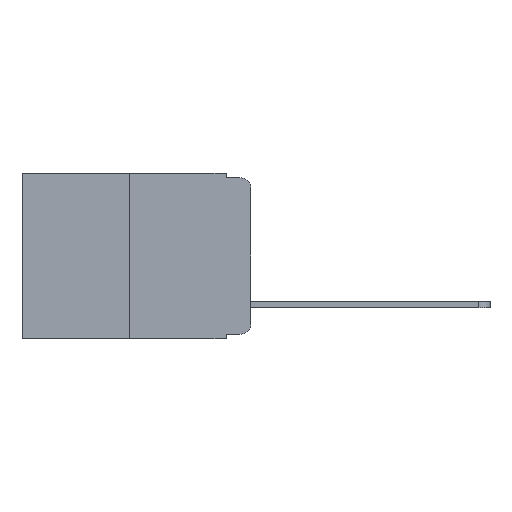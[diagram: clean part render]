
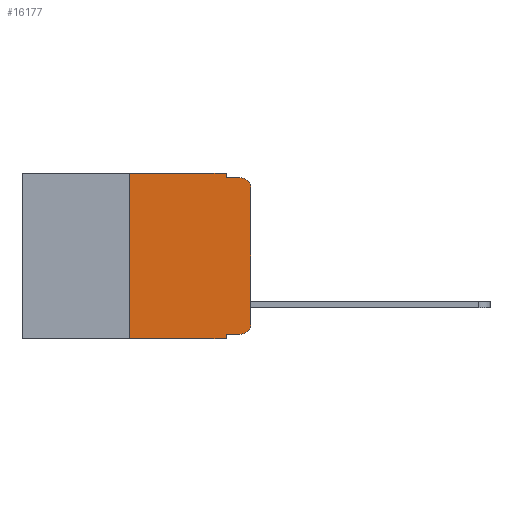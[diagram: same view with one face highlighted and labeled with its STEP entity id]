
A CAD part, left-side view. The second image highlights one B-rep face of the part: STEP entity #16177.
In plain terms, the highlighted planar face has unit normal (-1, 0, 0).
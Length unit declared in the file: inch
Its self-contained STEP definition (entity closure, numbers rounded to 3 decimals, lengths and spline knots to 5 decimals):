
#381 = DIRECTION ( 'NONE',  ( 0., -1., 0. ) ) ;
#1298 = LINE ( 'NONE', #11117, #1922 ) ;
#1876 = VECTOR ( 'NONE', #25471, 39.37008 ) ;
#1922 = VECTOR ( 'NONE', #12966, 39.37008 ) ;
#3066 = DIRECTION ( 'NONE',  ( 0., 0., -1. ) ) ;
#3145 = CARTESIAN_POINT ( 'NONE',  ( 0., 0.02, -0.313 ) ) ;
#3162 = ORIENTED_EDGE ( 'NONE', *, *, #18410, .T. ) ;
#3527 = CARTESIAN_POINT ( 'NONE',  ( 0., 0.473, 0. ) ) ;
#3782 = CARTESIAN_POINT ( 'NONE',  ( 0., 0.051, -0.01 ) ) ;
#4241 = ORIENTED_EDGE ( 'NONE', *, *, #22553, .F. ) ;
#4274 = CARTESIAN_POINT ( 'NONE',  ( 0., 0., -0.313 ) ) ;
#4508 = VERTEX_POINT ( 'NONE', #16672 ) ;
#5679 = LINE ( 'NONE', #9997, #5983 ) ;
#5983 = VECTOR ( 'NONE', #12033, 39.37008 ) ;
#6054 = LINE ( 'NONE', #16431, #22130 ) ;
#6550 = ORIENTED_EDGE ( 'NONE', *, *, #18586, .F. ) ;
#6836 = EDGE_CURVE ( 'NONE', #21819, #19800, #9442, .T. ) ;
#7178 = CARTESIAN_POINT ( 'NONE',  ( 0., 0.02, -0.01 ) ) ;
#7381 = VERTEX_POINT ( 'NONE', #7178 ) ;
#7676 = VERTEX_POINT ( 'NONE', #13423 ) ;
#7685 = VERTEX_POINT ( 'NONE', #25169 ) ;
#7914 = EDGE_LOOP ( 'NONE', ( #20988, #16805, #23745, #6550, #9480, #4241, #24558, #19415, #18828, #3162 ) ) ;
#8549 = CIRCLE ( 'NONE', #22609, 0.02 ) ;
#8832 = CARTESIAN_POINT ( 'NONE',  ( 0., 0.02, -0.03 ) ) ;
#9442 = LINE ( 'NONE', #25559, #26167 ) ;
#9480 = ORIENTED_EDGE ( 'NONE', *, *, #9622, .F. ) ;
#9574 = CARTESIAN_POINT ( 'NONE',  ( 0., 0.051, 0. ) ) ;
#9622 = EDGE_CURVE ( 'NONE', #22339, #7676, #6054, .T. ) ;
#9995 = EDGE_CURVE ( 'NONE', #4508, #7685, #1298, .T. ) ;
#9997 = CARTESIAN_POINT ( 'NONE',  ( 0., 0., 0. ) ) ;
#10143 = EDGE_CURVE ( 'NONE', #10325, #7381, #13927, .T. ) ;
#10325 = VERTEX_POINT ( 'NONE', #11975 ) ;
#10834 = DIRECTION ( 'NONE',  ( 0., 0., -1. ) ) ;
#11117 = CARTESIAN_POINT ( 'NONE',  ( 0., 0.051, -0.333 ) ) ;
#11201 = CARTESIAN_POINT ( 'NONE',  ( 0., 0.25, 0. ) ) ;
#11374 = LINE ( 'NONE', #9574, #1876 ) ;
#11426 = AXIS2_PLACEMENT_3D ( 'NONE', #3527, #21588, #15346 ) ;
#11616 = DIRECTION ( 'NONE',  ( 0., -1., 0. ) ) ;
#11975 = CARTESIAN_POINT ( 'NONE',  ( 0., 0., -0.03 ) ) ;
#12033 = DIRECTION ( 'NONE',  ( 0., 0., 1. ) ) ;
#12966 = DIRECTION ( 'NONE',  ( 0., -1., 0. ) ) ;
#12997 = AXIS2_PLACEMENT_3D ( 'NONE', #8832, #22926, #10834 ) ;
#13423 = CARTESIAN_POINT ( 'NONE',  ( 0., 0.051, 0. ) ) ;
#13927 = CIRCLE ( 'NONE', #12997, 0.02 ) ;
#14305 = CARTESIAN_POINT ( 'NONE',  ( 0., 0.051, -0.01 ) ) ;
#15310 = FACE_OUTER_BOUND ( 'NONE', #7914, .T. ) ;
#15346 = DIRECTION ( 'NONE',  ( 0., 0., -1. ) ) ;
#15600 = DIRECTION ( 'NONE',  ( 0., -1., 0. ) ) ;
#15630 = VERTEX_POINT ( 'NONE', #14305 ) ;
#16177 = ADVANCED_FACE ( 'NONE', ( #15310 ), #23552, .F. ) ;
#16303 = DIRECTION ( 'NONE',  ( 0., 0., -1. ) ) ;
#16431 = CARTESIAN_POINT ( 'NONE',  ( 0., 0.473, 0. ) ) ;
#16433 = LINE ( 'NONE', #3782, #21165 ) ;
#16484 = CARTESIAN_POINT ( 'NONE',  ( 0., 0.25, 0. ) ) ;
#16672 = CARTESIAN_POINT ( 'NONE',  ( 0., 0.051, -0.333 ) ) ;
#16805 = ORIENTED_EDGE ( 'NONE', *, *, #10143, .T. ) ;
#17286 = DIRECTION ( 'NONE',  ( 0., 0., 1. ) ) ;
#18088 = EDGE_CURVE ( 'NONE', #15630, #7381, #16433, .T. ) ;
#18410 = EDGE_CURVE ( 'NONE', #7685, #20173, #8549, .T. ) ;
#18415 = CARTESIAN_POINT ( 'NONE',  ( 0., 0.051, 0. ) ) ;
#18493 = LINE ( 'NONE', #18415, #23250 ) ;
#18586 = EDGE_CURVE ( 'NONE', #7676, #15630, #11374, .T. ) ;
#18703 = EDGE_CURVE ( 'NONE', #20173, #10325, #5679, .T. ) ;
#18828 = ORIENTED_EDGE ( 'NONE', *, *, #9995, .T. ) ;
#19192 = DIRECTION ( 'NONE',  ( -1., 0., 0. ) ) ;
#19415 = ORIENTED_EDGE ( 'NONE', *, *, #22396, .F. ) ;
#19466 = VECTOR ( 'NONE', #17286, 39.37008 ) ;
#19800 = VERTEX_POINT ( 'NONE', #24944 ) ;
#20173 = VERTEX_POINT ( 'NONE', #4274 ) ;
#20988 = ORIENTED_EDGE ( 'NONE', *, *, #18703, .T. ) ;
#21165 = VECTOR ( 'NONE', #15600, 39.37008 ) ;
#21588 = DIRECTION ( 'NONE',  ( 1., 0., 0. ) ) ;
#21819 = VERTEX_POINT ( 'NONE', #25818 ) ;
#22130 = VECTOR ( 'NONE', #381, 39.37008 ) ;
#22339 = VERTEX_POINT ( 'NONE', #16484 ) ;
#22396 = EDGE_CURVE ( 'NONE', #4508, #19800, #18493, .T. ) ;
#22553 = EDGE_CURVE ( 'NONE', #21819, #22339, #24847, .T. ) ;
#22609 = AXIS2_PLACEMENT_3D ( 'NONE', #3145, #19192, #3066 ) ;
#22926 = DIRECTION ( 'NONE',  ( -1., 0., 0. ) ) ;
#23250 = VECTOR ( 'NONE', #16303, 39.37008 ) ;
#23552 = PLANE ( 'NONE',  #11426 ) ;
#23745 = ORIENTED_EDGE ( 'NONE', *, *, #18088, .F. ) ;
#24558 = ORIENTED_EDGE ( 'NONE', *, *, #6836, .T. ) ;
#24847 = LINE ( 'NONE', #11201, #19466 ) ;
#24944 = CARTESIAN_POINT ( 'NONE',  ( 0., 0.051, -0.343 ) ) ;
#25169 = CARTESIAN_POINT ( 'NONE',  ( 0., 0.02, -0.333 ) ) ;
#25471 = DIRECTION ( 'NONE',  ( 0., 0., -1. ) ) ;
#25559 = CARTESIAN_POINT ( 'NONE',  ( 0., 0.473, -0.343 ) ) ;
#25818 = CARTESIAN_POINT ( 'NONE',  ( 0., 0.25, -0.343 ) ) ;
#26167 = VECTOR ( 'NONE', #11616, 39.37008 ) ;
